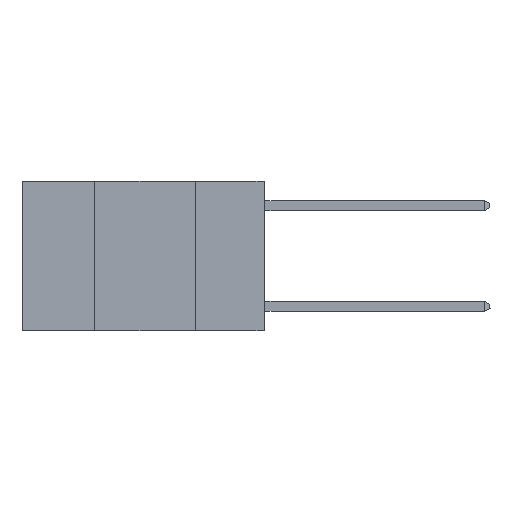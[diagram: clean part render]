
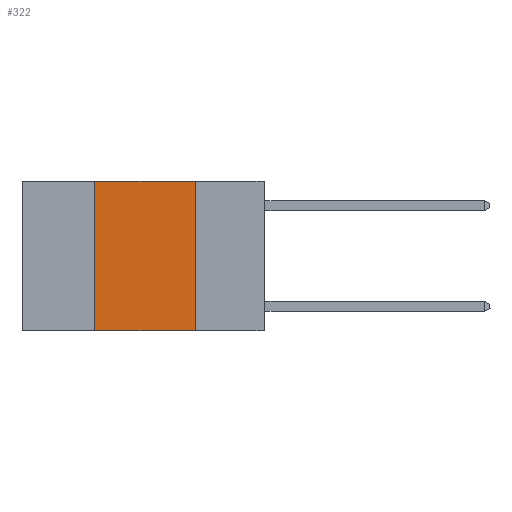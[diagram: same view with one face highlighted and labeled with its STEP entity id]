
A CAD part, left-side view. The second image highlights one B-rep face of the part: STEP entity #322.
In plain terms, the highlighted planar face has unit normal (-1, 0, 0).
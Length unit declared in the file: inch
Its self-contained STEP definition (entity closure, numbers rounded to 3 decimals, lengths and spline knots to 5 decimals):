
#322 = ADVANCED_FACE ( 'NONE', ( #4598 ), #3753, .F. ) ;
#371 = VERTEX_POINT ( 'NONE', #4783 ) ;
#788 = EDGE_CURVE ( 'NONE', #371, #5692, #1960, .T. ) ;
#813 = CARTESIAN_POINT ( 'NONE',  ( 0., 0.42, 0. ) ) ;
#1475 = ORIENTED_EDGE ( 'NONE', *, *, #788, .F. ) ;
#1571 = CARTESIAN_POINT ( 'NONE',  ( 0., 0.6, 0. ) ) ;
#1801 = ORIENTED_EDGE ( 'NONE', *, *, #4176, .F. ) ;
#1960 = LINE ( 'NONE', #9059, #9843 ) ;
#2845 = LINE ( 'NONE', #10454, #12751 ) ;
#2876 = EDGE_CURVE ( 'NONE', #5009, #5692, #10251, .T. ) ;
#2899 = DIRECTION ( 'NONE',  ( 0., 0., -1. ) ) ;
#2941 = DIRECTION ( 'NONE',  ( 0., 0., -1. ) ) ;
#3366 = DIRECTION ( 'NONE',  ( 0., -1., 0. ) ) ;
#3753 = PLANE ( 'NONE',  #4768 ) ;
#3847 = VECTOR ( 'NONE', #3366, 39.37008 ) ;
#4132 = ORIENTED_EDGE ( 'NONE', *, *, #6470, .F. ) ;
#4176 = EDGE_CURVE ( 'NONE', #5009, #8096, #2845, .T. ) ;
#4598 = FACE_OUTER_BOUND ( 'NONE', #11396, .T. ) ;
#4768 = AXIS2_PLACEMENT_3D ( 'NONE', #1571, #9427, #2899 ) ;
#4783 = CARTESIAN_POINT ( 'NONE',  ( 0., 0.17, 0. ) ) ;
#4924 = CARTESIAN_POINT ( 'NONE',  ( 0., 0.17, -0.37 ) ) ;
#5009 = VERTEX_POINT ( 'NONE', #6833 ) ;
#5294 = CARTESIAN_POINT ( 'NONE',  ( 0., 0.6, 0. ) ) ;
#5692 = VERTEX_POINT ( 'NONE', #4924 ) ;
#6457 = LINE ( 'NONE', #5294, #3847 ) ;
#6470 = EDGE_CURVE ( 'NONE', #8096, #371, #6457, .T. ) ;
#6487 = DIRECTION ( 'NONE',  ( 0., 0., 1. ) ) ;
#6833 = CARTESIAN_POINT ( 'NONE',  ( 0., 0.42, -0.37 ) ) ;
#7620 = VECTOR ( 'NONE', #12343, 39.37008 ) ;
#8096 = VERTEX_POINT ( 'NONE', #813 ) ;
#9059 = CARTESIAN_POINT ( 'NONE',  ( 0., 0.17, 0. ) ) ;
#9427 = DIRECTION ( 'NONE',  ( 1., 0., 0. ) ) ;
#9843 = VECTOR ( 'NONE', #2941, 39.37008 ) ;
#10251 = LINE ( 'NONE', #10277, #7620 ) ;
#10277 = CARTESIAN_POINT ( 'NONE',  ( 0., 0.6, -0.37 ) ) ;
#10454 = CARTESIAN_POINT ( 'NONE',  ( 0., 0.42, 0. ) ) ;
#11396 = EDGE_LOOP ( 'NONE', ( #1475, #4132, #1801, #12359 ) ) ;
#12343 = DIRECTION ( 'NONE',  ( 0., -1., 0. ) ) ;
#12359 = ORIENTED_EDGE ( 'NONE', *, *, #2876, .T. ) ;
#12751 = VECTOR ( 'NONE', #6487, 39.37008 ) ;
